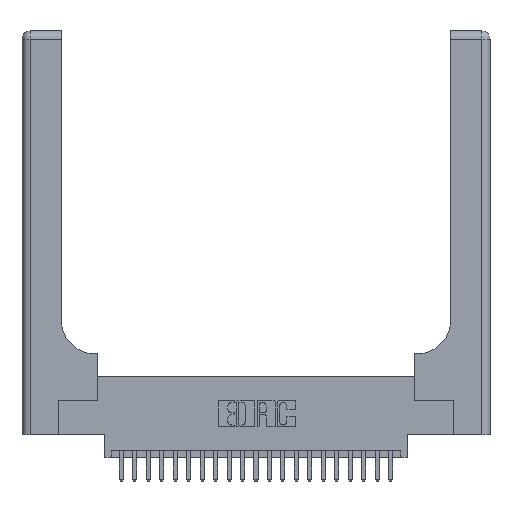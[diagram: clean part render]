
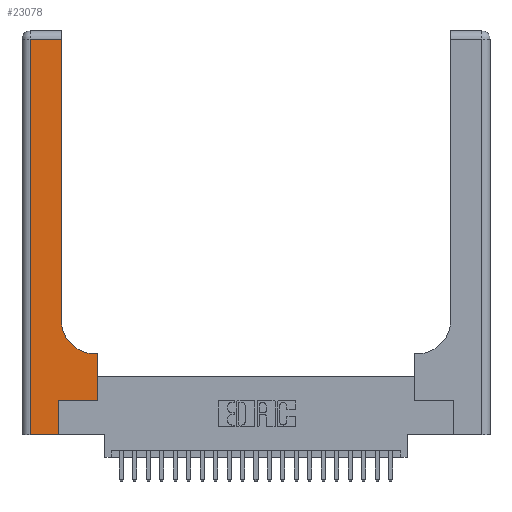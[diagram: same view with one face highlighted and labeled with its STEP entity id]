
A CAD part, top view. The second image highlights one B-rep face of the part: STEP entity #23078.
In plain terms, the highlighted planar face has unit normal (0, 0, 1).
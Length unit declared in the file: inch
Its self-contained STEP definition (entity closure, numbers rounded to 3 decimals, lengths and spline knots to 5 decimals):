
#180 = ORIENTED_EDGE ( 'NONE', *, *, #11288, .T. ) ;
#409 = ORIENTED_EDGE ( 'NONE', *, *, #20678, .T. ) ;
#505 = VERTEX_POINT ( 'NONE', #15640 ) ;
#1757 = AXIS2_PLACEMENT_3D ( 'NONE', #12746, #14648, #3205 ) ;
#1954 = VECTOR ( 'NONE', #8503, 39.37008 ) ;
#2876 = VERTEX_POINT ( 'NONE', #7144 ) ;
#3034 = EDGE_CURVE ( 'NONE', #6982, #23622, #7338, .T. ) ;
#3205 = DIRECTION ( 'NONE',  ( -1., 0., 0. ) ) ;
#3608 = VECTOR ( 'NONE', #19145, 39.37008 ) ;
#3856 = VECTOR ( 'NONE', #23058, 39.37008 ) ;
#4291 = VERTEX_POINT ( 'NONE', #13250 ) ;
#4368 = VERTEX_POINT ( 'NONE', #5756 ) ;
#4463 = VERTEX_POINT ( 'NONE', #15553 ) ;
#4893 = VERTEX_POINT ( 'NONE', #17113 ) ;
#5756 = CARTESIAN_POINT ( 'NONE',  ( 0.269, 0.25, 0.37 ) ) ;
#5832 = CARTESIAN_POINT ( 'NONE',  ( 0.269, 0., 0.37 ) ) ;
#5847 = LINE ( 'NONE', #5832, #15943 ) ;
#5857 = CARTESIAN_POINT ( 'NONE',  ( 0.269, 0.25, 0.37 ) ) ;
#6982 = VERTEX_POINT ( 'NONE', #23587 ) ;
#7102 = LINE ( 'NONE', #19859, #1954 ) ;
#7144 = CARTESIAN_POINT ( 'NONE',  ( 0.06, 2.94, 0.37 ) ) ;
#7267 = DIRECTION ( 'NONE',  ( 0., 1., 0. ) ) ;
#7338 = LINE ( 'NONE', #18929, #21867 ) ;
#7730 = FACE_OUTER_BOUND ( 'NONE', #9744, .T. ) ;
#8266 = ORIENTED_EDGE ( 'NONE', *, *, #19815, .T. ) ;
#8503 = DIRECTION ( 'NONE',  ( 0., 1., 0. ) ) ;
#8826 = CARTESIAN_POINT ( 'NONE',  ( 0.5415, 0.6, 0.37 ) ) ;
#8835 = EDGE_CURVE ( 'NONE', #4463, #4291, #17472, .T. ) ;
#9127 = DIRECTION ( 'NONE',  ( 0., 0., -1. ) ) ;
#9255 = CARTESIAN_POINT ( 'NONE',  ( 0.2915, 3., 0.37 ) ) ;
#9290 = CARTESIAN_POINT ( 'NONE',  ( 0., 2.94, 0.37 ) ) ;
#9744 = EDGE_LOOP ( 'NONE', ( #9986, #409, #8266, #21316, #13773, #180, #21143, #15972, #22401 ) ) ;
#9815 = CARTESIAN_POINT ( 'NONE',  ( 0., 0., 0.37 ) ) ;
#9986 = ORIENTED_EDGE ( 'NONE', *, *, #8835, .T. ) ;
#11288 = EDGE_CURVE ( 'NONE', #4368, #4893, #14360, .T. ) ;
#12204 = LINE ( 'NONE', #9815, #3856 ) ;
#12746 = CARTESIAN_POINT ( 'NONE',  ( 0., 3., 0.37 ) ) ;
#13006 = AXIS2_PLACEMENT_3D ( 'NONE', #20482, #9127, #22376 ) ;
#13250 = CARTESIAN_POINT ( 'NONE',  ( 0.2915, 2.94, 0.37 ) ) ;
#13773 = ORIENTED_EDGE ( 'NONE', *, *, #18643, .T. ) ;
#13811 = LINE ( 'NONE', #18739, #17666 ) ;
#13986 = CIRCLE ( 'NONE', #13006, 0.25 ) ;
#14349 = VECTOR ( 'NONE', #22219, 39.37008 ) ;
#14360 = LINE ( 'NONE', #5857, #3608 ) ;
#14648 = DIRECTION ( 'NONE',  ( 0., 0., -1. ) ) ;
#14952 = LINE ( 'NONE', #9290, #14349 ) ;
#15553 = CARTESIAN_POINT ( 'NONE',  ( 0.2915, 0.85, 0.37 ) ) ;
#15640 = CARTESIAN_POINT ( 'NONE',  ( 0.06, 0., 0.37 ) ) ;
#15943 = VECTOR ( 'NONE', #17210, 39.37008 ) ;
#15972 = ORIENTED_EDGE ( 'NONE', *, *, #3034, .T. ) ;
#17016 = DIRECTION ( 'NONE',  ( -1., 0., 0. ) ) ;
#17113 = CARTESIAN_POINT ( 'NONE',  ( 0.5585, 0.25, 0.37 ) ) ;
#17184 = EDGE_CURVE ( 'NONE', #4893, #6982, #7102, .T. ) ;
#17210 = DIRECTION ( 'NONE',  ( 0., 1., 0. ) ) ;
#17472 = LINE ( 'NONE', #9255, #18061 ) ;
#17666 = VECTOR ( 'NONE', #22546, 39.37008 ) ;
#18061 = VECTOR ( 'NONE', #7267, 39.37008 ) ;
#18643 = EDGE_CURVE ( 'NONE', #22911, #4368, #5847, .T. ) ;
#18739 = CARTESIAN_POINT ( 'NONE',  ( 0.06, 3., 0.37 ) ) ;
#18929 = CARTESIAN_POINT ( 'NONE',  ( 0.2915, 0.6, 0.37 ) ) ;
#19145 = DIRECTION ( 'NONE',  ( 1., 0., 0. ) ) ;
#19815 = EDGE_CURVE ( 'NONE', #2876, #505, #13811, .T. ) ;
#19859 = CARTESIAN_POINT ( 'NONE',  ( 0.5585, 0.25, 0.37 ) ) ;
#19881 = CARTESIAN_POINT ( 'NONE',  ( 0.269, 0., 0.37 ) ) ;
#20482 = CARTESIAN_POINT ( 'NONE',  ( 0.5415, 0.85, 0.37 ) ) ;
#20678 = EDGE_CURVE ( 'NONE', #4291, #2876, #14952, .T. ) ;
#21143 = ORIENTED_EDGE ( 'NONE', *, *, #17184, .T. ) ;
#21316 = ORIENTED_EDGE ( 'NONE', *, *, #22163, .T. ) ;
#21867 = VECTOR ( 'NONE', #17016, 39.37008 ) ;
#22163 = EDGE_CURVE ( 'NONE', #505, #22911, #12204, .T. ) ;
#22219 = DIRECTION ( 'NONE',  ( -1., 0., 0. ) ) ;
#22376 = DIRECTION ( 'NONE',  ( 1., 0., 0. ) ) ;
#22401 = ORIENTED_EDGE ( 'NONE', *, *, #22541, .T. ) ;
#22541 = EDGE_CURVE ( 'NONE', #23622, #4463, #13986, .T. ) ;
#22546 = DIRECTION ( 'NONE',  ( 0., -1., 0. ) ) ;
#22911 = VERTEX_POINT ( 'NONE', #19881 ) ;
#23058 = DIRECTION ( 'NONE',  ( 1., 0., 0. ) ) ;
#23078 = ADVANCED_FACE ( 'NONE', ( #7730 ), #24085, .F. ) ;
#23587 = CARTESIAN_POINT ( 'NONE',  ( 0.5585, 0.6, 0.37 ) ) ;
#23622 = VERTEX_POINT ( 'NONE', #8826 ) ;
#24085 = PLANE ( 'NONE',  #1757 ) ;
